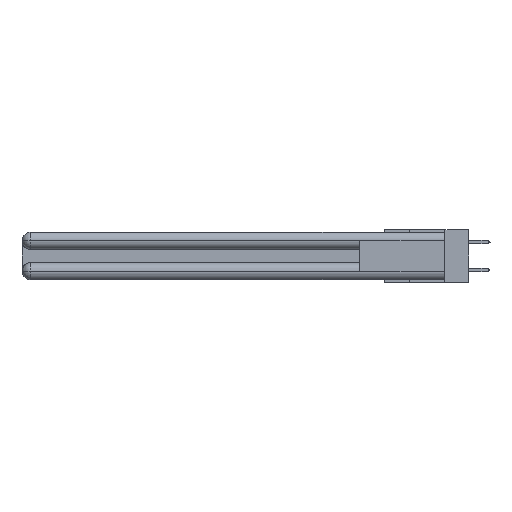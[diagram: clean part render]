
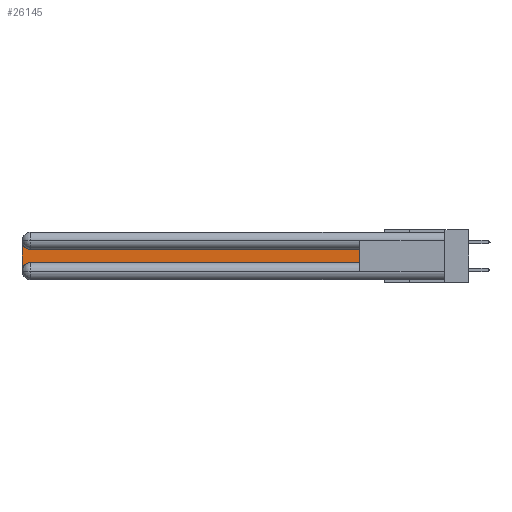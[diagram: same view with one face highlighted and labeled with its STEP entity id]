
A CAD part, left-side view. The second image highlights one B-rep face of the part: STEP entity #26145.
In plain terms, the highlighted planar face has unit normal (-1, 0, 0).
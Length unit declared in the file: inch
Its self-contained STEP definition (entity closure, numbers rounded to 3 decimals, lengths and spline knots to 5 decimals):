
#188 = AXIS2_PLACEMENT_3D ( 'NONE', #5951, #15195, #19581 ) ;
#1465 = LINE ( 'NONE', #6213, #21001 ) ;
#1513 = CARTESIAN_POINT ( 'NONE',  ( 0.075, 0.6, -0.1225 ) ) ;
#1852 = LINE ( 'NONE', #20570, #17588 ) ;
#2075 = VERTEX_POINT ( 'NONE', #11934 ) ;
#2092 = CARTESIAN_POINT ( 'NONE',  ( 0.075, 2.94, -0.2775 ) ) ;
#2189 = ORIENTED_EDGE ( 'NONE', *, *, #27069, .T. ) ;
#3533 = CARTESIAN_POINT ( 'NONE',  ( 0.075, 3., -0.0625 ) ) ;
#4192 = VECTOR ( 'NONE', #26361, 39.37008 ) ;
#5445 = ORIENTED_EDGE ( 'NONE', *, *, #15160, .T. ) ;
#5626 = ORIENTED_EDGE ( 'NONE', *, *, #11000, .T. ) ;
#5951 = CARTESIAN_POINT ( 'NONE',  ( 0.075, 3., -0.1225 ) ) ;
#6007 = VERTEX_POINT ( 'NONE', #19220 ) ;
#6202 = EDGE_CURVE ( 'NONE', #2075, #17138, #18198, .T. ) ;
#6213 = CARTESIAN_POINT ( 'NONE',  ( 0.075, 0.6, -0.2175 ) ) ;
#6439 = CIRCLE ( 'NONE', #6563, 0.06 ) ;
#6563 = AXIS2_PLACEMENT_3D ( 'NONE', #2092, #8856, #24415 ) ;
#7390 = VECTOR ( 'NONE', #24075, 39.37008 ) ;
#7786 = VERTEX_POINT ( 'NONE', #15178 ) ;
#8856 = DIRECTION ( 'NONE',  ( 1., 0., 0. ) ) ;
#9991 = EDGE_CURVE ( 'NONE', #10464, #16672, #13043, .T. ) ;
#10420 = CARTESIAN_POINT ( 'NONE',  ( 0.075, 0.6, -0.2175 ) ) ;
#10464 = VERTEX_POINT ( 'NONE', #18541 ) ;
#11000 = EDGE_CURVE ( 'NONE', #17138, #6007, #1465, .T. ) ;
#11934 = CARTESIAN_POINT ( 'NONE',  ( 0.075, 2.94, -0.2175 ) ) ;
#13043 = CIRCLE ( 'NONE', #28447, 0.06 ) ;
#13648 = LINE ( 'NONE', #1513, #4192 ) ;
#14559 = PLANE ( 'NONE',  #188 ) ;
#15110 = CARTESIAN_POINT ( 'NONE',  ( 0.075, 0.6, -0.2175 ) ) ;
#15160 = EDGE_CURVE ( 'NONE', #6007, #10464, #13648, .T. ) ;
#15178 = CARTESIAN_POINT ( 'NONE',  ( 0.075, 3., -0.2775 ) ) ;
#15195 = DIRECTION ( 'NONE',  ( 1., 0., 0. ) ) ;
#16470 = DIRECTION ( 'NONE',  ( 0., 0., -1. ) ) ;
#16672 = VERTEX_POINT ( 'NONE', #3533 ) ;
#17138 = VERTEX_POINT ( 'NONE', #10420 ) ;
#17556 = DIRECTION ( 'NONE',  ( 1., 0., 0. ) ) ;
#17588 = VECTOR ( 'NONE', #16470, 39.37008 ) ;
#17724 = DIRECTION ( 'NONE',  ( 0., 0., 1. ) ) ;
#18198 = LINE ( 'NONE', #15110, #7390 ) ;
#18541 = CARTESIAN_POINT ( 'NONE',  ( 0.075, 2.94, -0.1225 ) ) ;
#19220 = CARTESIAN_POINT ( 'NONE',  ( 0.075, 0.6, -0.1225 ) ) ;
#19581 = DIRECTION ( 'NONE',  ( 0., 0., -1. ) ) ;
#19675 = DIRECTION ( 'NONE',  ( 0., 0., -1. ) ) ;
#20570 = CARTESIAN_POINT ( 'NONE',  ( 0.075, 3., -0.2175 ) ) ;
#21001 = VECTOR ( 'NONE', #17724, 39.37008 ) ;
#21351 = ORIENTED_EDGE ( 'NONE', *, *, #26203, .T. ) ;
#21406 = FACE_OUTER_BOUND ( 'NONE', #26153, .T. ) ;
#24075 = DIRECTION ( 'NONE',  ( 0., -1., 0. ) ) ;
#24415 = DIRECTION ( 'NONE',  ( 0., 0., -1. ) ) ;
#26073 = ORIENTED_EDGE ( 'NONE', *, *, #9991, .T. ) ;
#26104 = CARTESIAN_POINT ( 'NONE',  ( 0.075, 2.94, -0.0625 ) ) ;
#26145 = ADVANCED_FACE ( 'NONE', ( #21406 ), #14559, .F. ) ;
#26153 = EDGE_LOOP ( 'NONE', ( #5445, #26073, #21351, #2189, #27610, #5626 ) ) ;
#26203 = EDGE_CURVE ( 'NONE', #16672, #7786, #1852, .T. ) ;
#26361 = DIRECTION ( 'NONE',  ( 0., 1., 0. ) ) ;
#27069 = EDGE_CURVE ( 'NONE', #7786, #2075, #6439, .T. ) ;
#27610 = ORIENTED_EDGE ( 'NONE', *, *, #6202, .T. ) ;
#28447 = AXIS2_PLACEMENT_3D ( 'NONE', #26104, #17556, #19675 ) ;
